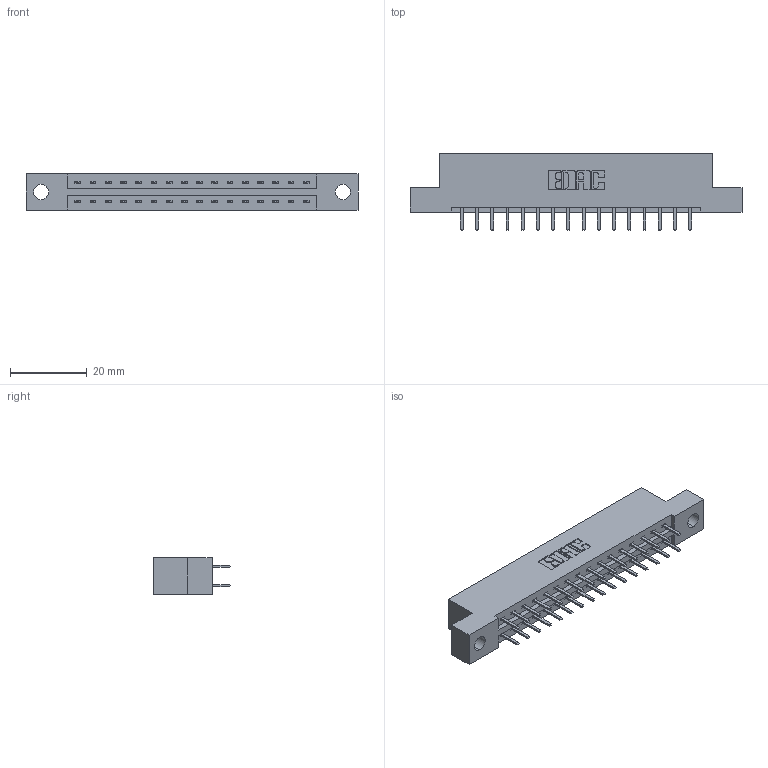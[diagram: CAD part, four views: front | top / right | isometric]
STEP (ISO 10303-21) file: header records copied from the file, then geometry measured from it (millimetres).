
FILE_DESCRIPTION (( 'STEP AP203' ), '1' );
FILE_NAME ('387-032-520-204.STEP', '2018-09-18T05:29:24', ( '' ), ( '' ), 'SwSTEP 2.0', 'SolidWorks 2016', '' );
FILE_SCHEMA (( 'CONFIG_CONTROL_DESIGN' ));
Length unit declared in the file: inch
Products named in the file (3): 337 Part_Flush Mounting Lugs - 0.156 Dia-TH; 345-292-001_345-293-120; 387-032-520-204
Assembly tree (33 placements, depth 2):
  387-032-520-204
    337 Part_Flush Mounting Lugs - 0.156 Dia-TH
    345-292-001_345-293-120  x32
Bounding box: 86.41 x 20.02 x 9.4 mm (x, y, z)
Volume: 8658.6 mm3; surface area: 9293.3 mm2
Topology: 33 solids, 33 shells, 1970 faces, 5719 edges, 3726 vertices
Faces by surface type: plane 1350, cylinder 620
Entity records: 15885 total; most frequent: CARTESIAN_POINT 2710, ORIENTED_EDGE 2634, DIRECTION 2341, EDGE_CURVE 1317, VECTOR 1185, LINE 1185, VERTEX_POINT 874, AXIS2_PLACEMENT_3D 578
